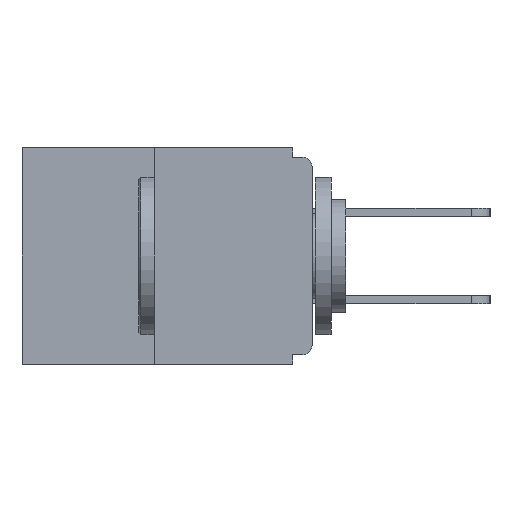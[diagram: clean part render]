
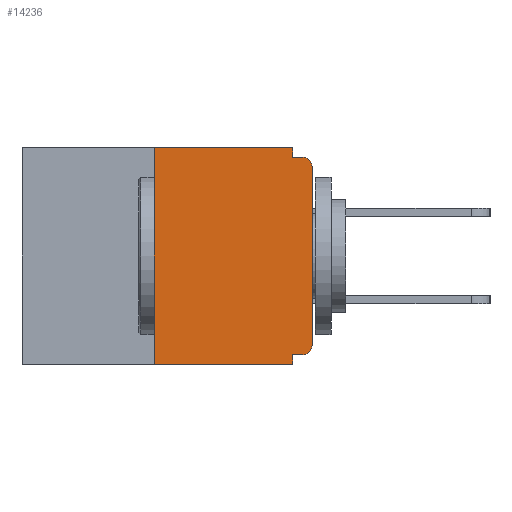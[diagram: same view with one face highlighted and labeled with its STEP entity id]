
A CAD part, left-side view. The second image highlights one B-rep face of the part: STEP entity #14236.
In plain terms, the highlighted planar face has unit normal (-1, 0, 0).
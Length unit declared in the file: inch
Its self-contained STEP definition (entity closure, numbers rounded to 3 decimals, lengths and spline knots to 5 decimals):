
#42 = CARTESIAN_POINT ( 'NONE',  ( 0., 0.031, -0.343 ) ) ;
#78 = CARTESIAN_POINT ( 'NONE',  ( 0., 0.25, -0.343 ) ) ;
#363 = VECTOR ( 'NONE', #7183, 39.37008 ) ;
#368 = CARTESIAN_POINT ( 'NONE',  ( 0., 0.031, 0. ) ) ;
#651 = CARTESIAN_POINT ( 'NONE',  ( 0., 0., -0.03 ) ) ;
#804 = EDGE_CURVE ( 'NONE', #15762, #6567, #12468, .T. ) ;
#928 = EDGE_CURVE ( 'NONE', #14248, #9867, #12804, .T. ) ;
#977 = ORIENTED_EDGE ( 'NONE', *, *, #6147, .T. ) ;
#1227 = DIRECTION ( 'NONE',  ( 0., -1., 0. ) ) ;
#1561 = CARTESIAN_POINT ( 'NONE',  ( 0., 0.031, -0.015 ) ) ;
#1563 = DIRECTION ( 'NONE',  ( 0., 0., -1. ) ) ;
#1673 = ORIENTED_EDGE ( 'NONE', *, *, #10559, .F. ) ;
#2071 = DIRECTION ( 'NONE',  ( 1., 0., 0. ) ) ;
#2397 = DIRECTION ( 'NONE',  ( 0., 0., -1. ) ) ;
#2563 = EDGE_CURVE ( 'NONE', #12493, #4716, #5277, .T. ) ;
#3182 = CARTESIAN_POINT ( 'NONE',  ( 0., 0.031, -0.328 ) ) ;
#3254 = EDGE_CURVE ( 'NONE', #10052, #11201, #13294, .T. ) ;
#3789 = CARTESIAN_POINT ( 'NONE',  ( 0., 0., -0.313 ) ) ;
#4298 = DIRECTION ( 'NONE',  ( 0., -1., 0. ) ) ;
#4317 = CARTESIAN_POINT ( 'NONE',  ( 0., 0.031, 0. ) ) ;
#4413 = VERTEX_POINT ( 'NONE', #78 ) ;
#4496 = CARTESIAN_POINT ( 'NONE',  ( 0., 0.015, -0.328 ) ) ;
#4716 = VERTEX_POINT ( 'NONE', #6741 ) ;
#4759 = LINE ( 'NONE', #8237, #363 ) ;
#4957 = LINE ( 'NONE', #368, #9381 ) ;
#5223 = ORIENTED_EDGE ( 'NONE', *, *, #3254, .F. ) ;
#5277 = LINE ( 'NONE', #13956, #13123 ) ;
#5387 = CARTESIAN_POINT ( 'NONE',  ( 0., 0.25, 0. ) ) ;
#5710 = DIRECTION ( 'NONE',  ( 0., 1., 0. ) ) ;
#6147 = EDGE_CURVE ( 'NONE', #8924, #4716, #9614, .T. ) ;
#6150 = AXIS2_PLACEMENT_3D ( 'NONE', #13319, #9648, #2397 ) ;
#6567 = VERTEX_POINT ( 'NONE', #4317 ) ;
#6633 = CARTESIAN_POINT ( 'NONE',  ( 0., 0., 0. ) ) ;
#6741 = CARTESIAN_POINT ( 'NONE',  ( 0., 0.015, -0.015 ) ) ;
#6858 = ORIENTED_EDGE ( 'NONE', *, *, #7940, .F. ) ;
#7011 = LINE ( 'NONE', #6633, #12563 ) ;
#7183 = DIRECTION ( 'NONE',  ( 0., -1., 0. ) ) ;
#7571 = ORIENTED_EDGE ( 'NONE', *, *, #8161, .F. ) ;
#7906 = AXIS2_PLACEMENT_3D ( 'NONE', #15610, #2071, #15501 ) ;
#7940 = EDGE_CURVE ( 'NONE', #6567, #12493, #4957, .T. ) ;
#8085 = DIRECTION ( 'NONE',  ( 0., 0., -1. ) ) ;
#8106 = PLANE ( 'NONE',  #7906 ) ;
#8161 = EDGE_CURVE ( 'NONE', #4413, #15762, #12792, .T. ) ;
#8237 = CARTESIAN_POINT ( 'NONE',  ( 0., 0.46, -0.343 ) ) ;
#8317 = EDGE_CURVE ( 'NONE', #4413, #11201, #4759, .T. ) ;
#8376 = ORIENTED_EDGE ( 'NONE', *, *, #928, .T. ) ;
#8571 = CARTESIAN_POINT ( 'NONE',  ( 0., 0.25, 0. ) ) ;
#8924 = VERTEX_POINT ( 'NONE', #651 ) ;
#8964 = ORIENTED_EDGE ( 'NONE', *, *, #8317, .T. ) ;
#9177 = FACE_OUTER_BOUND ( 'NONE', #10749, .T. ) ;
#9197 = VECTOR ( 'NONE', #1227, 39.37008 ) ;
#9381 = VECTOR ( 'NONE', #1563, 39.37008 ) ;
#9488 = LINE ( 'NONE', #15278, #13862 ) ;
#9614 = CIRCLE ( 'NONE', #6150, 0.015 ) ;
#9618 = EDGE_CURVE ( 'NONE', #9867, #8924, #7011, .T. ) ;
#9648 = DIRECTION ( 'NONE',  ( -1., 0., 0. ) ) ;
#9867 = VERTEX_POINT ( 'NONE', #3789 ) ;
#10052 = VERTEX_POINT ( 'NONE', #3182 ) ;
#10357 = DIRECTION ( 'NONE',  ( 0., 0., 1. ) ) ;
#10559 = EDGE_CURVE ( 'NONE', #14248, #10052, #9488, .T. ) ;
#10749 = EDGE_LOOP ( 'NONE', ( #12596, #7571, #8964, #5223, #1673, #8376, #14991, #977, #15507, #6858 ) ) ;
#11201 = VERTEX_POINT ( 'NONE', #42 ) ;
#12325 = CARTESIAN_POINT ( 'NONE',  ( 0., 0.46, 0. ) ) ;
#12365 = DIRECTION ( 'NONE',  ( 0., 0., 1. ) ) ;
#12468 = LINE ( 'NONE', #12325, #9197 ) ;
#12493 = VERTEX_POINT ( 'NONE', #1561 ) ;
#12563 = VECTOR ( 'NONE', #10357, 39.37008 ) ;
#12596 = ORIENTED_EDGE ( 'NONE', *, *, #804, .F. ) ;
#12792 = LINE ( 'NONE', #8571, #13166 ) ;
#12804 = CIRCLE ( 'NONE', #15117, 0.015 ) ;
#13005 = CARTESIAN_POINT ( 'NONE',  ( 0., 0.031, -0.343 ) ) ;
#13123 = VECTOR ( 'NONE', #4298, 39.37008 ) ;
#13166 = VECTOR ( 'NONE', #12365, 39.37008 ) ;
#13294 = LINE ( 'NONE', #13005, #14241 ) ;
#13319 = CARTESIAN_POINT ( 'NONE',  ( 0., 0.015, -0.03 ) ) ;
#13862 = VECTOR ( 'NONE', #5710, 39.37008 ) ;
#13956 = CARTESIAN_POINT ( 'NONE',  ( 0., 0., -0.015 ) ) ;
#14140 = CARTESIAN_POINT ( 'NONE',  ( 0., 0.015, -0.313 ) ) ;
#14236 = ADVANCED_FACE ( 'NONE', ( #9177 ), #8106, .F. ) ;
#14241 = VECTOR ( 'NONE', #15290, 39.37008 ) ;
#14248 = VERTEX_POINT ( 'NONE', #4496 ) ;
#14298 = DIRECTION ( 'NONE',  ( -1., 0., 0. ) ) ;
#14991 = ORIENTED_EDGE ( 'NONE', *, *, #9618, .T. ) ;
#15117 = AXIS2_PLACEMENT_3D ( 'NONE', #14140, #14298, #8085 ) ;
#15278 = CARTESIAN_POINT ( 'NONE',  ( 0., 0., -0.328 ) ) ;
#15290 = DIRECTION ( 'NONE',  ( 0., 0., -1. ) ) ;
#15501 = DIRECTION ( 'NONE',  ( 0., 0., -1. ) ) ;
#15507 = ORIENTED_EDGE ( 'NONE', *, *, #2563, .F. ) ;
#15610 = CARTESIAN_POINT ( 'NONE',  ( 0., 0.46, 0. ) ) ;
#15762 = VERTEX_POINT ( 'NONE', #5387 ) ;
